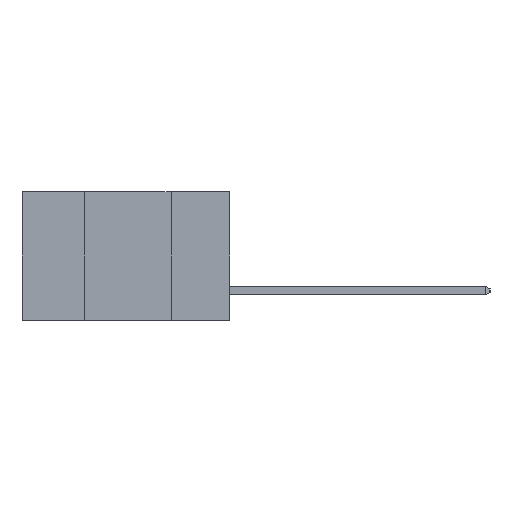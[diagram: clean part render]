
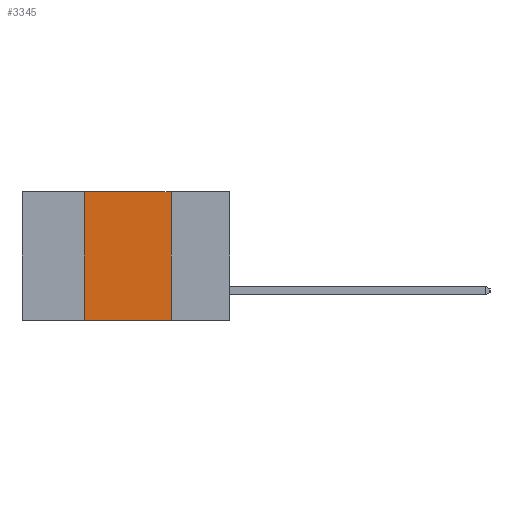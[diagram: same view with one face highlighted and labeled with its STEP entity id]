
A CAD part, left-side view. The second image highlights one B-rep face of the part: STEP entity #3345.
In plain terms, the highlighted planar face has unit normal (-1, 0, 0).
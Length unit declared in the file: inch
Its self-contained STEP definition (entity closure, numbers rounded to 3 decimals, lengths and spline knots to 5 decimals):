
#1325 = VERTEX_POINT ( 'NONE', #3442 ) ;
#1505 = DIRECTION ( 'NONE',  ( 0., -1., 0. ) ) ;
#2179 = EDGE_CURVE ( 'NONE', #11889, #7722, #15843, .T. ) ;
#2191 = PLANE ( 'NONE',  #15863 ) ;
#2710 = ORIENTED_EDGE ( 'NONE', *, *, #3082, .F. ) ;
#3082 = EDGE_CURVE ( 'NONE', #11889, #3573, #7514, .T. ) ;
#3216 = CARTESIAN_POINT ( 'NONE',  ( 0., 0.42, -0.37 ) ) ;
#3345 = ADVANCED_FACE ( 'NONE', ( #9053 ), #2191, .F. ) ;
#3442 = CARTESIAN_POINT ( 'NONE',  ( 0., 0.17, 0. ) ) ;
#3469 = CARTESIAN_POINT ( 'NONE',  ( 0., 0.6, 0. ) ) ;
#3554 = ORIENTED_EDGE ( 'NONE', *, *, #3968, .F. ) ;
#3573 = VERTEX_POINT ( 'NONE', #4876 ) ;
#3968 = EDGE_CURVE ( 'NONE', #1325, #7722, #15031, .T. ) ;
#4876 = CARTESIAN_POINT ( 'NONE',  ( 0., 0.42, 0. ) ) ;
#5059 = CARTESIAN_POINT ( 'NONE',  ( 0., 0.17, 0. ) ) ;
#5405 = DIRECTION ( 'NONE',  ( 0., 0., -1. ) ) ;
#5487 = VECTOR ( 'NONE', #5405, 39.37008 ) ;
#6186 = ORIENTED_EDGE ( 'NONE', *, *, #15740, .F. ) ;
#7128 = VECTOR ( 'NONE', #10859, 39.37008 ) ;
#7514 = LINE ( 'NONE', #9820, #7128 ) ;
#7673 = LINE ( 'NONE', #11420, #8089 ) ;
#7722 = VERTEX_POINT ( 'NONE', #9459 ) ;
#7905 = CARTESIAN_POINT ( 'NONE',  ( 0., 0.6, -0.37 ) ) ;
#8089 = VECTOR ( 'NONE', #11364, 39.37008 ) ;
#9053 = FACE_OUTER_BOUND ( 'NONE', #11178, .T. ) ;
#9459 = CARTESIAN_POINT ( 'NONE',  ( 0., 0.17, -0.37 ) ) ;
#9820 = CARTESIAN_POINT ( 'NONE',  ( 0., 0.42, 0. ) ) ;
#9831 = DIRECTION ( 'NONE',  ( 0., 0., -1. ) ) ;
#10859 = DIRECTION ( 'NONE',  ( 0., 0., 1. ) ) ;
#11178 = EDGE_LOOP ( 'NONE', ( #3554, #6186, #2710, #13199 ) ) ;
#11364 = DIRECTION ( 'NONE',  ( 0., -1., 0. ) ) ;
#11420 = CARTESIAN_POINT ( 'NONE',  ( 0., 0.6, 0. ) ) ;
#11889 = VERTEX_POINT ( 'NONE', #3216 ) ;
#12905 = VECTOR ( 'NONE', #1505, 39.37008 ) ;
#13199 = ORIENTED_EDGE ( 'NONE', *, *, #2179, .T. ) ;
#13767 = DIRECTION ( 'NONE',  ( 1., 0., 0. ) ) ;
#15031 = LINE ( 'NONE', #5059, #5487 ) ;
#15740 = EDGE_CURVE ( 'NONE', #3573, #1325, #7673, .T. ) ;
#15843 = LINE ( 'NONE', #7905, #12905 ) ;
#15863 = AXIS2_PLACEMENT_3D ( 'NONE', #3469, #13767, #9831 ) ;
